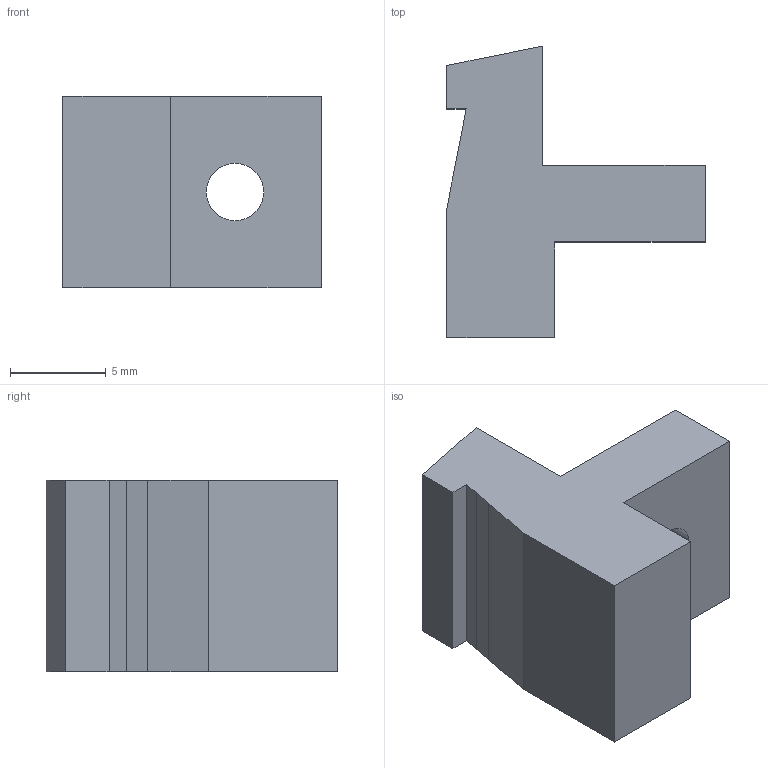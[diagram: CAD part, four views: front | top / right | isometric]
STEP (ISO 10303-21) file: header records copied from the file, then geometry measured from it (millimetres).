
FILE_DESCRIPTION (( 'STEP AP203' ), '1' );
FILE_NAME ('MOD9_feed_ramp.STEP', '2020-06-10T04:59:11', ( '' ), ( '' ), 'SwSTEP 2.0', 'SolidWorks 2016', '' );
FILE_SCHEMA (( 'CONFIG_CONTROL_DESIGN' ));
Length unit declared in the file: millimetre
Products named in the file (1): MOD9_feed_ramp
Bounding box: 13.5 x 15.24 x 10 mm (x, y, z)
Volume: 1026.5 mm3; surface area: 810.9 mm2
Topology: 1 solids, 1 shells, 18 faces, 47 edges, 31 vertices
Faces by surface type: plane 16, cone 1, cylinder 1
Full cylindrical faces by diameter (mm): 3 x1
Entity records: 617 total; most frequent: CARTESIAN_POINT 95, ORIENTED_EDGE 90, DIRECTION 86, EDGE_CURVE 45, VECTOR 42, LINE 42, VERTEX_POINT 31, EDGE_LOOP 22
